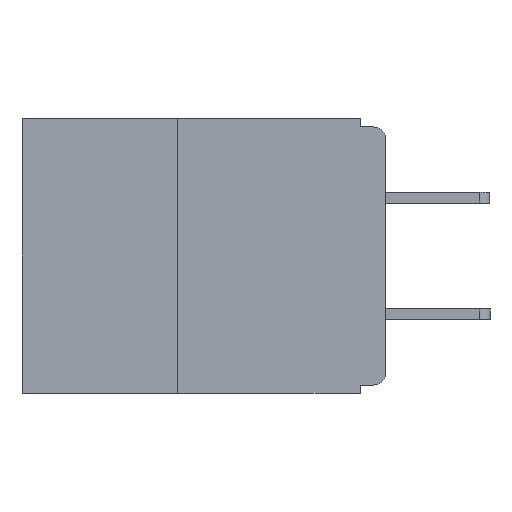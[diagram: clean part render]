
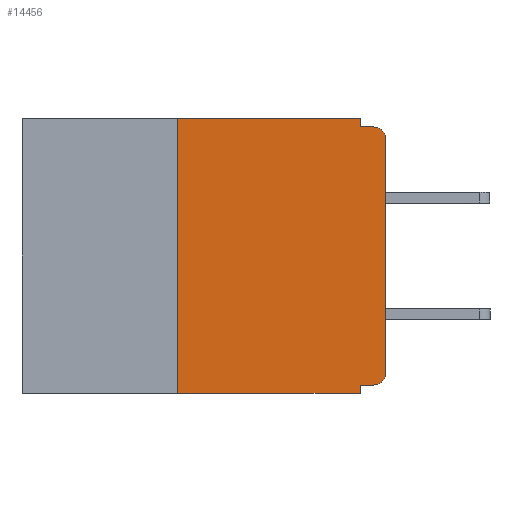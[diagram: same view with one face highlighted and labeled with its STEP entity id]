
A CAD part, left-side view. The second image highlights one B-rep face of the part: STEP entity #14456.
In plain terms, the highlighted planar face has unit normal (-1, 0, 0).
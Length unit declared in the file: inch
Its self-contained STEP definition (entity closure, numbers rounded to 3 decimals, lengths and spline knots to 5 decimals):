
#336 = DIRECTION ( 'NONE',  ( 0., 0., -1. ) ) ;
#486 = CARTESIAN_POINT ( 'NONE',  ( 0., 0.031, -0.33 ) ) ;
#772 = VERTEX_POINT ( 'NONE', #16364 ) ;
#962 = CARTESIAN_POINT ( 'NONE',  ( 0., 0.015, -0.32 ) ) ;
#1115 = CARTESIAN_POINT ( 'NONE',  ( 0., 0., -0.305 ) ) ;
#1341 = LINE ( 'NONE', #14335, #11797 ) ;
#1400 = CARTESIAN_POINT ( 'NONE',  ( 0., 0.015, -0.025 ) ) ;
#1968 = VERTEX_POINT ( 'NONE', #1115 ) ;
#2366 = AXIS2_PLACEMENT_3D ( 'NONE', #1400, #14249, #3276 ) ;
#2712 = VECTOR ( 'NONE', #336, 39.37008 ) ;
#2727 = ORIENTED_EDGE ( 'NONE', *, *, #9567, .F. ) ;
#2927 = VERTEX_POINT ( 'NONE', #18167 ) ;
#3276 = DIRECTION ( 'NONE',  ( 0., 0., -1. ) ) ;
#3945 = VERTEX_POINT ( 'NONE', #8185 ) ;
#4480 = ORIENTED_EDGE ( 'NONE', *, *, #22136, .F. ) ;
#4623 = LINE ( 'NONE', #6142, #14906 ) ;
#4847 = VERTEX_POINT ( 'NONE', #17763 ) ;
#4985 = EDGE_CURVE ( 'NONE', #4847, #2927, #7319, .T. ) ;
#5578 = DIRECTION ( 'NONE',  ( 0., -1., 0. ) ) ;
#5943 = ORIENTED_EDGE ( 'NONE', *, *, #4985, .F. ) ;
#6142 = CARTESIAN_POINT ( 'NONE',  ( 0., 0., -0.32 ) ) ;
#7319 = LINE ( 'NONE', #13384, #12221 ) ;
#7584 = CIRCLE ( 'NONE', #13284, 0.015 ) ;
#7644 = CARTESIAN_POINT ( 'NONE',  ( 0., 0.437, 0. ) ) ;
#7728 = DIRECTION ( 'NONE',  ( 0., -1., 0. ) ) ;
#8185 = CARTESIAN_POINT ( 'NONE',  ( 0., 0.031, 0. ) ) ;
#8544 = CARTESIAN_POINT ( 'NONE',  ( 0., 0.031, -0.32 ) ) ;
#8742 = DIRECTION ( 'NONE',  ( 1., 0., 0. ) ) ;
#8906 = CARTESIAN_POINT ( 'NONE',  ( 0., 0.25, -0.33 ) ) ;
#9408 = CARTESIAN_POINT ( 'NONE',  ( 0., 0.015, -0.305 ) ) ;
#9567 = EDGE_CURVE ( 'NONE', #11028, #3945, #13129, .T. ) ;
#9622 = LINE ( 'NONE', #486, #23041 ) ;
#9752 = DIRECTION ( 'NONE',  ( 0., 0., -1. ) ) ;
#10595 = ORIENTED_EDGE ( 'NONE', *, *, #14028, .T. ) ;
#11028 = VERTEX_POINT ( 'NONE', #19011 ) ;
#11215 = EDGE_CURVE ( 'NONE', #1968, #11652, #1341, .T. ) ;
#11292 = DIRECTION ( 'NONE',  ( 0., 0., -1. ) ) ;
#11652 = VERTEX_POINT ( 'NONE', #22452 ) ;
#11760 = CARTESIAN_POINT ( 'NONE',  ( 0., 0.031, -0.33 ) ) ;
#11797 = VECTOR ( 'NONE', #12563, 39.37008 ) ;
#12175 = LINE ( 'NONE', #21509, #20877 ) ;
#12221 = VECTOR ( 'NONE', #13340, 39.37008 ) ;
#12561 = ORIENTED_EDGE ( 'NONE', *, *, #16449, .F. ) ;
#12563 = DIRECTION ( 'NONE',  ( 0., 0., 1. ) ) ;
#12569 = VECTOR ( 'NONE', #7728, 39.37008 ) ;
#13026 = FACE_OUTER_BOUND ( 'NONE', #21647, .T. ) ;
#13129 = LINE ( 'NONE', #7644, #12569 ) ;
#13284 = AXIS2_PLACEMENT_3D ( 'NONE', #9408, #21705, #11292 ) ;
#13340 = DIRECTION ( 'NONE',  ( 0., -1., 0. ) ) ;
#13384 = CARTESIAN_POINT ( 'NONE',  ( 0., 0., -0.01 ) ) ;
#13659 = LINE ( 'NONE', #21864, #2712 ) ;
#13676 = ORIENTED_EDGE ( 'NONE', *, *, #14162, .F. ) ;
#13928 = ORIENTED_EDGE ( 'NONE', *, *, #11215, .T. ) ;
#14028 = EDGE_CURVE ( 'NONE', #16280, #1968, #7584, .T. ) ;
#14136 = CARTESIAN_POINT ( 'NONE',  ( 0., 0.437, 0. ) ) ;
#14162 = EDGE_CURVE ( 'NONE', #17385, #14210, #9622, .T. ) ;
#14210 = VERTEX_POINT ( 'NONE', #11760 ) ;
#14249 = DIRECTION ( 'NONE',  ( -1., 0., 0. ) ) ;
#14335 = CARTESIAN_POINT ( 'NONE',  ( 0., 0., 0. ) ) ;
#14456 = ADVANCED_FACE ( 'NONE', ( #13026 ), #19330, .F. ) ;
#14489 = ORIENTED_EDGE ( 'NONE', *, *, #17472, .T. ) ;
#14906 = VECTOR ( 'NONE', #18628, 39.37008 ) ;
#15313 = EDGE_CURVE ( 'NONE', #772, #14210, #12175, .T. ) ;
#15668 = CIRCLE ( 'NONE', #2366, 0.015 ) ;
#15693 = AXIS2_PLACEMENT_3D ( 'NONE', #14136, #8742, #21097 ) ;
#16280 = VERTEX_POINT ( 'NONE', #962 ) ;
#16364 = CARTESIAN_POINT ( 'NONE',  ( 0., 0.25, -0.33 ) ) ;
#16449 = EDGE_CURVE ( 'NONE', #772, #11028, #19441, .T. ) ;
#17385 = VERTEX_POINT ( 'NONE', #8544 ) ;
#17472 = EDGE_CURVE ( 'NONE', #11652, #2927, #15668, .T. ) ;
#17763 = CARTESIAN_POINT ( 'NONE',  ( 0., 0.031, -0.01 ) ) ;
#18167 = CARTESIAN_POINT ( 'NONE',  ( 0., 0.015, -0.01 ) ) ;
#18628 = DIRECTION ( 'NONE',  ( 0., 1., 0. ) ) ;
#19011 = CARTESIAN_POINT ( 'NONE',  ( 0., 0.25, 0. ) ) ;
#19330 = PLANE ( 'NONE',  #15693 ) ;
#19441 = LINE ( 'NONE', #8906, #20550 ) ;
#19960 = EDGE_CURVE ( 'NONE', #3945, #4847, #13659, .T. ) ;
#20550 = VECTOR ( 'NONE', #21245, 39.37008 ) ;
#20877 = VECTOR ( 'NONE', #5578, 39.37008 ) ;
#21097 = DIRECTION ( 'NONE',  ( 0., 0., -1. ) ) ;
#21245 = DIRECTION ( 'NONE',  ( 0., 0., 1. ) ) ;
#21246 = ORIENTED_EDGE ( 'NONE', *, *, #19960, .F. ) ;
#21509 = CARTESIAN_POINT ( 'NONE',  ( 0., 0.437, -0.33 ) ) ;
#21647 = EDGE_LOOP ( 'NONE', ( #13928, #14489, #5943, #21246, #2727, #12561, #21777, #13676, #4480, #10595 ) ) ;
#21705 = DIRECTION ( 'NONE',  ( -1., 0., 0. ) ) ;
#21777 = ORIENTED_EDGE ( 'NONE', *, *, #15313, .T. ) ;
#21864 = CARTESIAN_POINT ( 'NONE',  ( 0., 0.031, 0. ) ) ;
#22136 = EDGE_CURVE ( 'NONE', #16280, #17385, #4623, .T. ) ;
#22452 = CARTESIAN_POINT ( 'NONE',  ( 0., 0., -0.025 ) ) ;
#23041 = VECTOR ( 'NONE', #9752, 39.37008 ) ;
